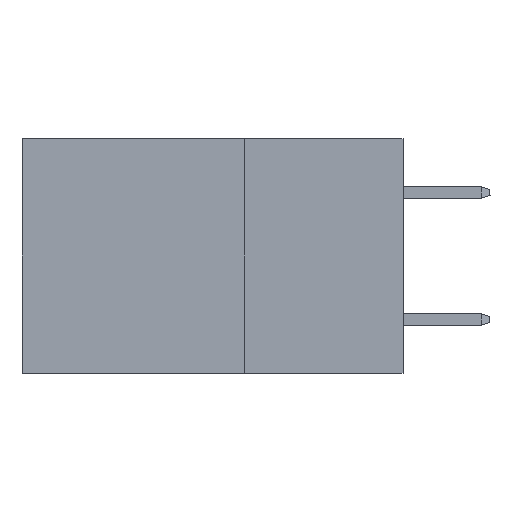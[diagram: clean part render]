
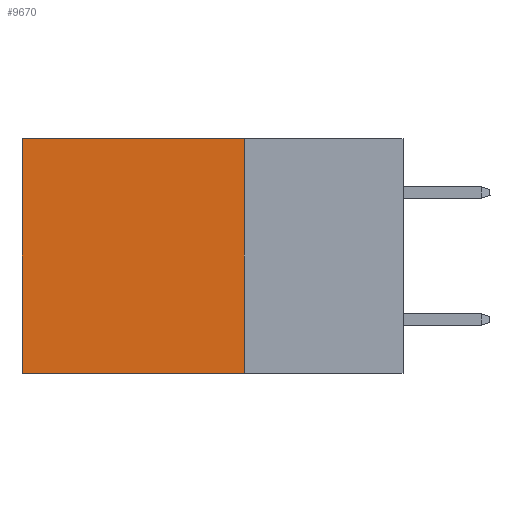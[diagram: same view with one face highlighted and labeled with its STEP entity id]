
A CAD part, left-side view. The second image highlights one B-rep face of the part: STEP entity #9670.
In plain terms, the highlighted planar face has unit normal (-1, 0, 0).
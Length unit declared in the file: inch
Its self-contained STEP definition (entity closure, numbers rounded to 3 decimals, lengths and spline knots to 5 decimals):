
#543 = EDGE_CURVE ( 'NONE', #14105, #15465, #10716, .T. ) ;
#7834 = ORIENTED_EDGE ( 'NONE', *, *, #29533, .T. ) ;
#7934 = CARTESIAN_POINT ( 'NONE',  ( 0.2875, 0.25, 0. ) ) ;
#8380 = CARTESIAN_POINT ( 'NONE',  ( 0.2875, 0.25, 0. ) ) ;
#8953 = ORIENTED_EDGE ( 'NONE', *, *, #543, .F. ) ;
#9005 = VECTOR ( 'NONE', #10343, 39.37008 ) ;
#9594 = ORIENTED_EDGE ( 'NONE', *, *, #12568, .F. ) ;
#9670 = ADVANCED_FACE ( 'NONE', ( #24928 ), #25086, .F. ) ;
#10343 = DIRECTION ( 'NONE',  ( 0., 1., 0. ) ) ;
#10659 = LINE ( 'NONE', #10821, #29479 ) ;
#10716 = LINE ( 'NONE', #8380, #11244 ) ;
#10821 = CARTESIAN_POINT ( 'NONE',  ( 0.2875, 0.6, 0. ) ) ;
#11244 = VECTOR ( 'NONE', #22144, 39.37008 ) ;
#12568 = EDGE_CURVE ( 'NONE', #15465, #27060, #24002, .T. ) ;
#13128 = DIRECTION ( 'NONE',  ( 0., 0., -1. ) ) ;
#13208 = DIRECTION ( 'NONE',  ( 0., 0., -1. ) ) ;
#14105 = VERTEX_POINT ( 'NONE', #7934 ) ;
#14550 = DIRECTION ( 'NONE',  ( 0., 1., 0. ) ) ;
#15465 = VERTEX_POINT ( 'NONE', #20386 ) ;
#15650 = CARTESIAN_POINT ( 'NONE',  ( 0.2875, 0.25, 0. ) ) ;
#17914 = LINE ( 'NONE', #29580, #9005 ) ;
#18010 = DIRECTION ( 'NONE',  ( 1., 0., 0. ) ) ;
#18182 = AXIS2_PLACEMENT_3D ( 'NONE', #15650, #18010, #13128 ) ;
#20386 = CARTESIAN_POINT ( 'NONE',  ( 0.2875, 0.25, -0.37 ) ) ;
#22144 = DIRECTION ( 'NONE',  ( 0., 0., -1. ) ) ;
#22661 = EDGE_CURVE ( 'NONE', #14105, #22697, #17914, .T. ) ;
#22697 = VERTEX_POINT ( 'NONE', #24840 ) ;
#23758 = VECTOR ( 'NONE', #14550, 39.37008 ) ;
#24002 = LINE ( 'NONE', #26069, #23758 ) ;
#24840 = CARTESIAN_POINT ( 'NONE',  ( 0.2875, 0.6, 0. ) ) ;
#24928 = FACE_OUTER_BOUND ( 'NONE', #28404, .T. ) ;
#25086 = PLANE ( 'NONE',  #18182 ) ;
#26069 = CARTESIAN_POINT ( 'NONE',  ( 0.2875, 0.25, -0.37 ) ) ;
#26682 = CARTESIAN_POINT ( 'NONE',  ( 0.2875, 0.6, -0.37 ) ) ;
#27060 = VERTEX_POINT ( 'NONE', #26682 ) ;
#28369 = ORIENTED_EDGE ( 'NONE', *, *, #22661, .T. ) ;
#28404 = EDGE_LOOP ( 'NONE', ( #7834, #9594, #8953, #28369 ) ) ;
#29479 = VECTOR ( 'NONE', #13208, 39.37008 ) ;
#29533 = EDGE_CURVE ( 'NONE', #22697, #27060, #10659, .T. ) ;
#29580 = CARTESIAN_POINT ( 'NONE',  ( 0.2875, 0.25, 0. ) ) ;
